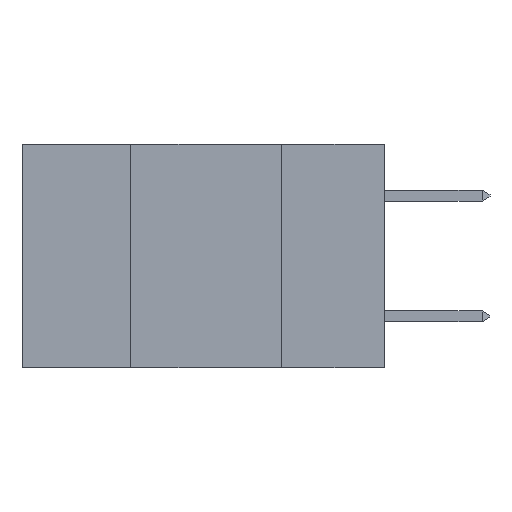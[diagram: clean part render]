
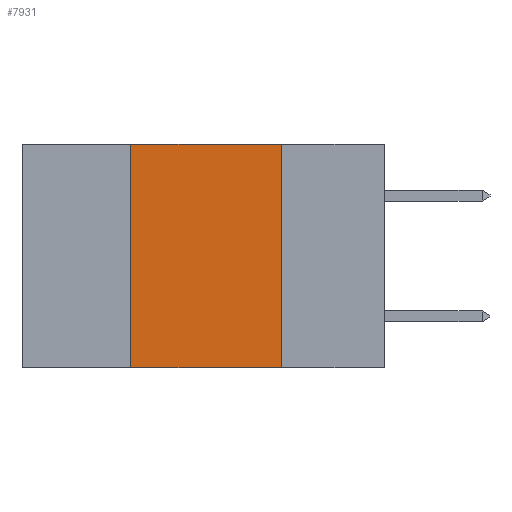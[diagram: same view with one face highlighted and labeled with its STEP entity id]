
A CAD part, left-side view. The second image highlights one B-rep face of the part: STEP entity #7931.
In plain terms, the highlighted planar face has unit normal (-1, 0, 0).
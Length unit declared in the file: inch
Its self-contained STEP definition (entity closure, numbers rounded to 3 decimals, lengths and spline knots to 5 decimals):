
#677 = EDGE_CURVE ( 'NONE', #9069, #2703, #7844, .T. ) ;
#940 = DIRECTION ( 'NONE',  ( 0., -1., 0. ) ) ;
#1164 = ORIENTED_EDGE ( 'NONE', *, *, #9080, .F. ) ;
#1748 = DIRECTION ( 'NONE',  ( 0., 0., -1. ) ) ;
#1752 = VERTEX_POINT ( 'NONE', #8328 ) ;
#1798 = CARTESIAN_POINT ( 'NONE',  ( 0., 0.6, 0. ) ) ;
#1960 = VECTOR ( 'NONE', #4713, 39.37008 ) ;
#2113 = DIRECTION ( 'NONE',  ( 1., 0., 0. ) ) ;
#2174 = FACE_OUTER_BOUND ( 'NONE', #3035, .T. ) ;
#2314 = CARTESIAN_POINT ( 'NONE',  ( 0., 0.17, 0. ) ) ;
#2703 = VERTEX_POINT ( 'NONE', #5053 ) ;
#2907 = ORIENTED_EDGE ( 'NONE', *, *, #8187, .F. ) ;
#3035 = EDGE_LOOP ( 'NONE', ( #2907, #4784, #1164, #3138 ) ) ;
#3138 = ORIENTED_EDGE ( 'NONE', *, *, #677, .T. ) ;
#3196 = CARTESIAN_POINT ( 'NONE',  ( 0., 0.17, 0. ) ) ;
#3557 = VERTEX_POINT ( 'NONE', #2314 ) ;
#3672 = VECTOR ( 'NONE', #4676, 39.37008 ) ;
#3990 = CARTESIAN_POINT ( 'NONE',  ( 0., 0.42, 0. ) ) ;
#4676 = DIRECTION ( 'NONE',  ( 0., -1., 0. ) ) ;
#4713 = DIRECTION ( 'NONE',  ( 0., 0., 1. ) ) ;
#4784 = ORIENTED_EDGE ( 'NONE', *, *, #9048, .F. ) ;
#4886 = VECTOR ( 'NONE', #1748, 39.37008 ) ;
#4936 = PLANE ( 'NONE',  #6624 ) ;
#5053 = CARTESIAN_POINT ( 'NONE',  ( 0., 0.17, -0.37 ) ) ;
#5514 = LINE ( 'NONE', #1798, #3672 ) ;
#5997 = VECTOR ( 'NONE', #940, 39.37008 ) ;
#6317 = CARTESIAN_POINT ( 'NONE',  ( 0., 0.6, 0. ) ) ;
#6624 = AXIS2_PLACEMENT_3D ( 'NONE', #6317, #2113, #7011 ) ;
#7011 = DIRECTION ( 'NONE',  ( 0., 0., -1. ) ) ;
#7119 = LINE ( 'NONE', #3990, #1960 ) ;
#7461 = CARTESIAN_POINT ( 'NONE',  ( 0., 0.42, -0.37 ) ) ;
#7844 = LINE ( 'NONE', #9081, #5997 ) ;
#7931 = ADVANCED_FACE ( 'NONE', ( #2174 ), #4936, .F. ) ;
#8187 = EDGE_CURVE ( 'NONE', #3557, #2703, #8531, .T. ) ;
#8328 = CARTESIAN_POINT ( 'NONE',  ( 0., 0.42, 0. ) ) ;
#8531 = LINE ( 'NONE', #3196, #4886 ) ;
#9048 = EDGE_CURVE ( 'NONE', #1752, #3557, #5514, .T. ) ;
#9069 = VERTEX_POINT ( 'NONE', #7461 ) ;
#9080 = EDGE_CURVE ( 'NONE', #9069, #1752, #7119, .T. ) ;
#9081 = CARTESIAN_POINT ( 'NONE',  ( 0., 0.6, -0.37 ) ) ;
